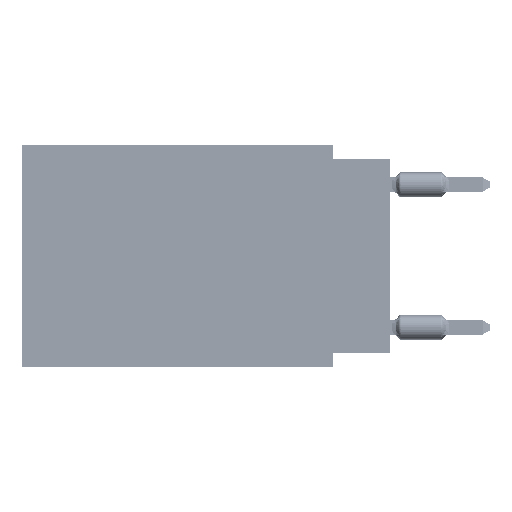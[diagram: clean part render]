
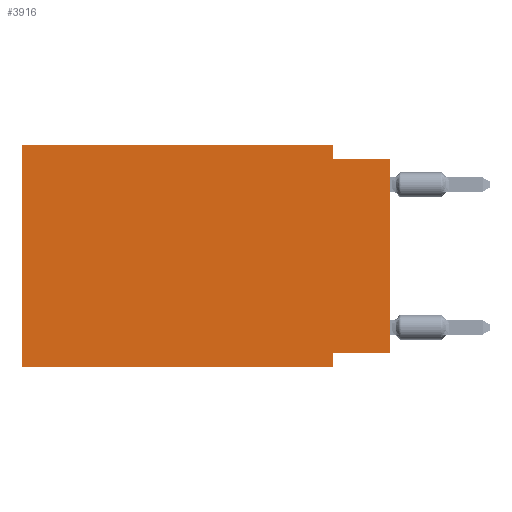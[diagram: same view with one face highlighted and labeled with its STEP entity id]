
A CAD part, left-side view. The second image highlights one B-rep face of the part: STEP entity #3916.
In plain terms, the highlighted planar face has unit normal (-1, 0, 0).
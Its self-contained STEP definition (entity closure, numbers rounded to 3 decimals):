
#1493 = ORIENTED_EDGE ( 'NONE', *, *, #79501, .F. ) ;
#1967 = VERTEX_POINT ( 'NONE', #40898 ) ;
#3916 = ADVANCED_FACE ( 'NONE', ( #32859 ), #45634, .F. ) ;
#3992 = CARTESIAN_POINT ( 'NONE',  ( 0., 16.383, 0. ) ) ;
#9017 = CARTESIAN_POINT ( 'NONE',  ( 0., 16.383, 0. ) ) ;
#9897 = ORIENTED_EDGE ( 'NONE', *, *, #27906, .T. ) ;
#10658 = VERTEX_POINT ( 'NONE', #53734 ) ;
#12014 = VERTEX_POINT ( 'NONE', #16602 ) ;
#12319 = LINE ( 'NONE', #31744, #26341 ) ;
#14253 = DIRECTION ( 'NONE',  ( 1., 0., 0. ) ) ;
#14486 = VECTOR ( 'NONE', #75683, 1000. ) ;
#14583 = ORIENTED_EDGE ( 'NONE', *, *, #80599, .F. ) ;
#16602 = CARTESIAN_POINT ( 'NONE',  ( 0., 2.54, -9.906 ) ) ;
#18190 = EDGE_CURVE ( 'NONE', #79503, #12014, #77961, .T. ) ;
#19600 = CARTESIAN_POINT ( 'NONE',  ( 0., 0., 0. ) ) ;
#21589 = ORIENTED_EDGE ( 'NONE', *, *, #18190, .T. ) ;
#23642 = VECTOR ( 'NONE', #79578, 1000. ) ;
#24332 = LINE ( 'NONE', #42508, #42402 ) ;
#25262 = AXIS2_PLACEMENT_3D ( 'NONE', #70783, #14253, #39458 ) ;
#25266 = DIRECTION ( 'NONE',  ( 0., -1., 0. ) ) ;
#25475 = EDGE_CURVE ( 'NONE', #74833, #1967, #73354, .T. ) ;
#26341 = VECTOR ( 'NONE', #37935, 1000. ) ;
#26678 = CARTESIAN_POINT ( 'NONE',  ( 0., 2.54, -9.271 ) ) ;
#27477 = ORIENTED_EDGE ( 'NONE', *, *, #68967, .F. ) ;
#27684 = LINE ( 'NONE', #76792, #52644 ) ;
#27883 = CARTESIAN_POINT ( 'NONE',  ( 0., 0., -9.271 ) ) ;
#27906 = EDGE_CURVE ( 'NONE', #62237, #62165, #56086, .T. ) ;
#28504 = ORIENTED_EDGE ( 'NONE', *, *, #61663, .F. ) ;
#31144 = CARTESIAN_POINT ( 'NONE',  ( 0., 2.54, 0. ) ) ;
#31744 = CARTESIAN_POINT ( 'NONE',  ( 0., 2.54, -9.906 ) ) ;
#32859 = FACE_OUTER_BOUND ( 'NONE', #72219, .T. ) ;
#36680 = CARTESIAN_POINT ( 'NONE',  ( 0., 0., -0.635 ) ) ;
#37935 = DIRECTION ( 'NONE',  ( 0., 0., -1. ) ) ;
#39245 = CARTESIAN_POINT ( 'NONE',  ( 0., 16.383, -9.906 ) ) ;
#39458 = DIRECTION ( 'NONE',  ( 0., 0., -1. ) ) ;
#40898 = CARTESIAN_POINT ( 'NONE',  ( 0., 2.54, 0. ) ) ;
#42402 = VECTOR ( 'NONE', #75094, 1000. ) ;
#42508 = CARTESIAN_POINT ( 'NONE',  ( 0., 0., -9.271 ) ) ;
#45634 = PLANE ( 'NONE',  #25262 ) ;
#52644 = VECTOR ( 'NONE', #52868, 1000. ) ;
#52868 = DIRECTION ( 'NONE',  ( 0., -1., 0. ) ) ;
#53722 = LINE ( 'NONE', #71859, #62976 ) ;
#53734 = CARTESIAN_POINT ( 'NONE',  ( 0., 2.54, -0.635 ) ) ;
#56086 = LINE ( 'NONE', #19600, #69762 ) ;
#57202 = VECTOR ( 'NONE', #25266, 1000. ) ;
#61663 = EDGE_CURVE ( 'NONE', #79503, #74833, #53722, .T. ) ;
#62165 = VERTEX_POINT ( 'NONE', #36680 ) ;
#62237 = VERTEX_POINT ( 'NONE', #27883 ) ;
#62976 = VECTOR ( 'NONE', #65691, 1000. ) ;
#65691 = DIRECTION ( 'NONE',  ( 0., 0., 1. ) ) ;
#67856 = LINE ( 'NONE', #31144, #14486 ) ;
#68967 = EDGE_CURVE ( 'NONE', #62237, #81614, #24332, .T. ) ;
#69738 = ORIENTED_EDGE ( 'NONE', *, *, #25475, .F. ) ;
#69762 = VECTOR ( 'NONE', #70362, 1000. ) ;
#70362 = DIRECTION ( 'NONE',  ( 0., 0., 1. ) ) ;
#70783 = CARTESIAN_POINT ( 'NONE',  ( 0., 16.383, 0. ) ) ;
#71859 = CARTESIAN_POINT ( 'NONE',  ( 0., 16.383, 0. ) ) ;
#72219 = EDGE_LOOP ( 'NONE', ( #9897, #1493, #14583, #69738, #28504, #21589, #81465, #27477 ) ) ;
#73354 = LINE ( 'NONE', #3992, #23642 ) ;
#74833 = VERTEX_POINT ( 'NONE', #9017 ) ;
#75094 = DIRECTION ( 'NONE',  ( 0., 1., 0. ) ) ;
#75594 = CARTESIAN_POINT ( 'NONE',  ( 0., 16.383, -9.906 ) ) ;
#75683 = DIRECTION ( 'NONE',  ( 0., 0., -1. ) ) ;
#76792 = CARTESIAN_POINT ( 'NONE',  ( 0., 0., -0.635 ) ) ;
#77961 = LINE ( 'NONE', #75594, #57202 ) ;
#79501 = EDGE_CURVE ( 'NONE', #10658, #62165, #27684, .T. ) ;
#79503 = VERTEX_POINT ( 'NONE', #39245 ) ;
#79578 = DIRECTION ( 'NONE',  ( 0., -1., 0. ) ) ;
#79835 = EDGE_CURVE ( 'NONE', #81614, #12014, #12319, .T. ) ;
#80599 = EDGE_CURVE ( 'NONE', #1967, #10658, #67856, .T. ) ;
#81465 = ORIENTED_EDGE ( 'NONE', *, *, #79835, .F. ) ;
#81614 = VERTEX_POINT ( 'NONE', #26678 ) ;
